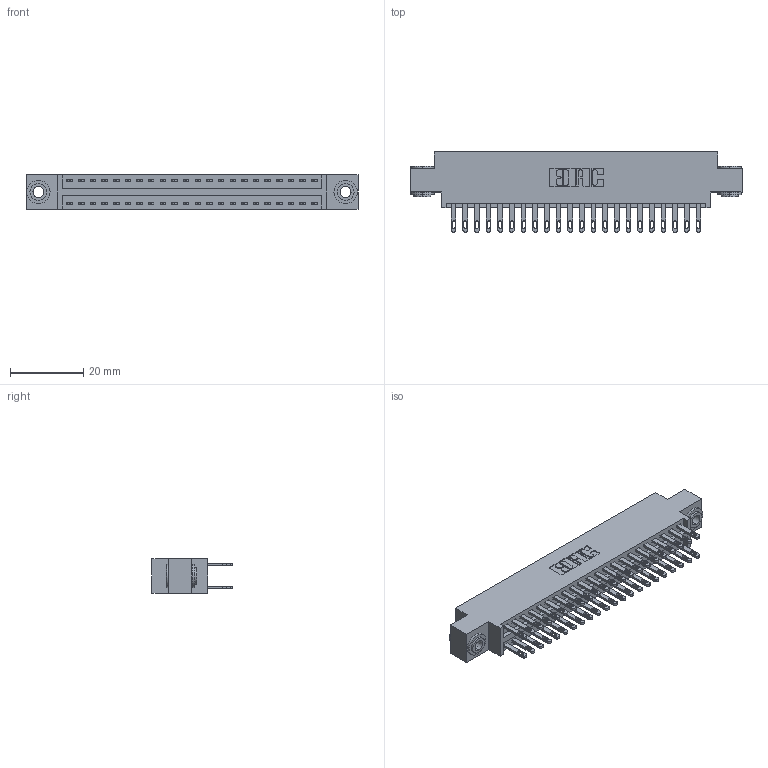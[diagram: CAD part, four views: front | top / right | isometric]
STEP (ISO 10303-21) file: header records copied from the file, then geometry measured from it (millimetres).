
FILE_DESCRIPTION (( 'STEP AP203' ), '1' );
FILE_NAME ('896-044-500-803.STEP', '2021-07-27T22:11:27', ( '' ), ( '' ), 'SwSTEP 2.0', 'SolidWorks 2020', '' );
FILE_SCHEMA (( 'CONFIG_CONTROL_DESIGN' ));
Length unit declared in the file: inch
Products named in the file (4): 345-292-001_345-293-100; 345-250-002_345-250-002-102; 846 Part_0.170 Offset - 0.156 Dia-TH; 896-044-500-803
Assembly tree (47 placements, depth 2):
  896-044-500-803
    846 Part_0.170 Offset - 0.156 Dia-TH
    345-292-001_345-293-100  x44
    345-250-002_345-250-002-102  x2
Bounding box: 90.42 x 21.84 x 9.4 mm (x, y, z)
Volume: 8661.4 mm3; surface area: 12445.6 mm2
Topology: 47 solids, 47 shells, 2276 faces, 6885 edges, 4586 vertices
Faces by surface type: plane 1366, cylinder 902, cone 8
Entity records: 17762 total; most frequent: CARTESIAN_POINT 2931, ORIENTED_EDGE 2858, DIRECTION 2667, EDGE_CURVE 1429, LINE 1181, VECTOR 1181, VERTEX_POINT 950, AXIS2_PLACEMENT_3D 743
